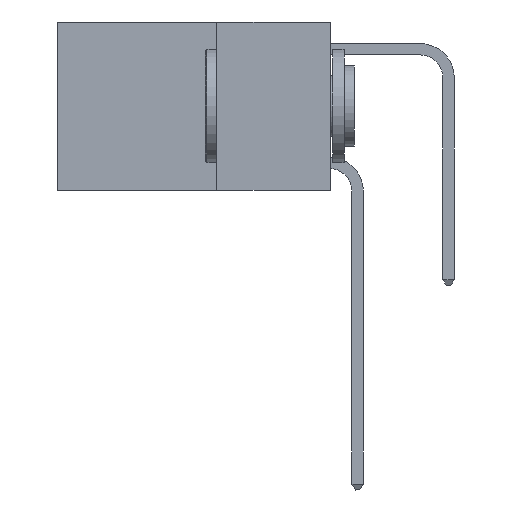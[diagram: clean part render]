
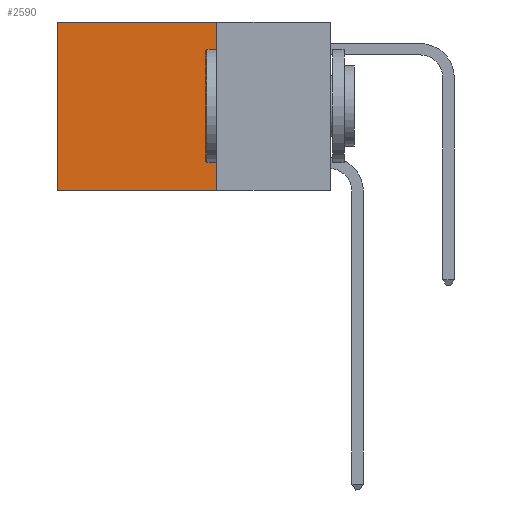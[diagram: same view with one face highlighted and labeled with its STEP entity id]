
A CAD part, left-side view. The second image highlights one B-rep face of the part: STEP entity #2590.
In plain terms, the highlighted planar face has unit normal (-1, 0, 0).
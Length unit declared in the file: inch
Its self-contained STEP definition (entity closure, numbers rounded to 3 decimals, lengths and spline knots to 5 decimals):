
#344 = LINE ( 'NONE', #18073, #20495 ) ;
#530 = LINE ( 'NONE', #20311, #12081 ) ;
#681 = ORIENTED_EDGE ( 'NONE', *, *, #11216, .F. ) ;
#1360 = ORIENTED_EDGE ( 'NONE', *, *, #13996, .F. ) ;
#1561 = DIRECTION ( 'NONE',  ( 0., 0., -1. ) ) ;
#1610 = EDGE_CURVE ( 'NONE', #16458, #10613, #6382, .T. ) ;
#1677 = CARTESIAN_POINT ( 'NONE',  ( 0.2625, 0.25, 0. ) ) ;
#2590 = ADVANCED_FACE ( 'NONE', ( #8268 ), #20905, .F. ) ;
#2911 = ORIENTED_EDGE ( 'NONE', *, *, #20639, .T. ) ;
#3754 = VERTEX_POINT ( 'NONE', #15397 ) ;
#4910 = CARTESIAN_POINT ( 'NONE',  ( 0.2625, 0.25, 0. ) ) ;
#5689 = DIRECTION ( 'NONE',  ( 0., 1., 0. ) ) ;
#6382 = LINE ( 'NONE', #8564, #18256 ) ;
#6397 = ORIENTED_EDGE ( 'NONE', *, *, #1610, .T. ) ;
#6611 = DIRECTION ( 'NONE',  ( 0., 1., 0. ) ) ;
#8268 = FACE_OUTER_BOUND ( 'NONE', #16969, .T. ) ;
#8492 = LINE ( 'NONE', #1677, #10904 ) ;
#8564 = CARTESIAN_POINT ( 'NONE',  ( 0.2625, 0.25, 0. ) ) ;
#9709 = CARTESIAN_POINT ( 'NONE',  ( 0.2625, 0.25, -0.37 ) ) ;
#10509 = DIRECTION ( 'NONE',  ( 0., 0., -1. ) ) ;
#10613 = VERTEX_POINT ( 'NONE', #13380 ) ;
#10904 = VECTOR ( 'NONE', #10509, 39.37008 ) ;
#11216 = EDGE_CURVE ( 'NONE', #16458, #16249, #8492, .T. ) ;
#12081 = VECTOR ( 'NONE', #22218, 39.37008 ) ;
#13380 = CARTESIAN_POINT ( 'NONE',  ( 0.2625, 0.6, 0. ) ) ;
#13996 = EDGE_CURVE ( 'NONE', #16249, #3754, #344, .T. ) ;
#15397 = CARTESIAN_POINT ( 'NONE',  ( 0.2625, 0.6, -0.37 ) ) ;
#15658 = AXIS2_PLACEMENT_3D ( 'NONE', #4910, #22793, #1561 ) ;
#16249 = VERTEX_POINT ( 'NONE', #9709 ) ;
#16458 = VERTEX_POINT ( 'NONE', #17889 ) ;
#16969 = EDGE_LOOP ( 'NONE', ( #2911, #1360, #681, #6397 ) ) ;
#17889 = CARTESIAN_POINT ( 'NONE',  ( 0.2625, 0.25, 0. ) ) ;
#18073 = CARTESIAN_POINT ( 'NONE',  ( 0.2625, 0.25, -0.37 ) ) ;
#18256 = VECTOR ( 'NONE', #6611, 39.37008 ) ;
#20311 = CARTESIAN_POINT ( 'NONE',  ( 0.2625, 0.6, 0. ) ) ;
#20495 = VECTOR ( 'NONE', #5689, 39.37008 ) ;
#20639 = EDGE_CURVE ( 'NONE', #10613, #3754, #530, .T. ) ;
#20905 = PLANE ( 'NONE',  #15658 ) ;
#22218 = DIRECTION ( 'NONE',  ( 0., 0., -1. ) ) ;
#22793 = DIRECTION ( 'NONE',  ( 1., 0., 0. ) ) ;
